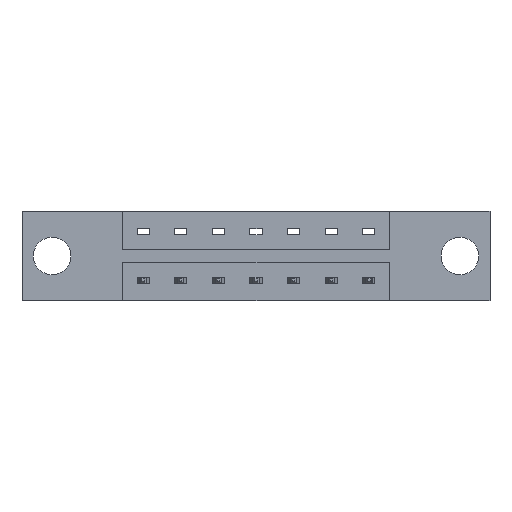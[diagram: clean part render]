
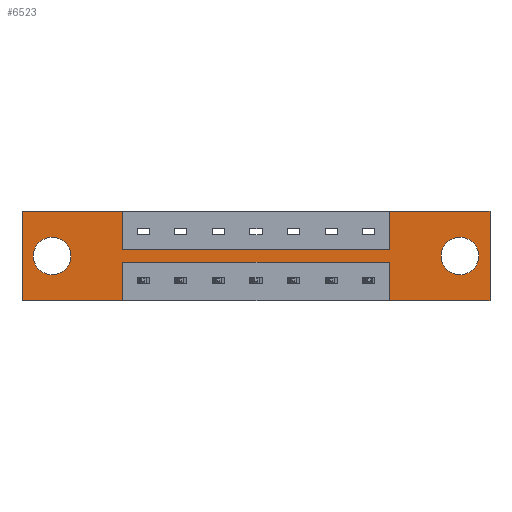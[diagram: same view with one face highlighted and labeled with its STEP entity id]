
A CAD part, front view. The second image highlights one B-rep face of the part: STEP entity #6523.
In plain terms, the highlighted planar face has unit normal (0, -1, 0).
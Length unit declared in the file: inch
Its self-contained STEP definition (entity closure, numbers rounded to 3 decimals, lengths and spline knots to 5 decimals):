
#17 = VECTOR ( 'NONE', #7473, 39.37008 ) ;
#23 = ORIENTED_EDGE ( 'NONE', *, *, #1032, .F. ) ;
#30 = ORIENTED_EDGE ( 'NONE', *, *, #563, .F. ) ;
#57 = ORIENTED_EDGE ( 'NONE', *, *, #378, .F. ) ;
#73 = ORIENTED_EDGE ( 'NONE', *, *, #656, .F. ) ;
#110 = ORIENTED_EDGE ( 'NONE', *, *, #6834, .T. ) ;
#120 = ORIENTED_EDGE ( 'NONE', *, *, #4638, .T. ) ;
#165 = ORIENTED_EDGE ( 'NONE', *, *, #4374, .T. ) ;
#191 = VECTOR ( 'NONE', #8565, 39.37008 ) ;
#202 = ORIENTED_EDGE ( 'NONE', *, *, #7367, .T. ) ;
#263 = LINE ( 'NONE', #601, #5720 ) ;
#378 = EDGE_CURVE ( 'NONE', #4003, #1568, #4932, .T. ) ;
#405 = DIRECTION ( 'NONE',  ( -1., 0., 0. ) ) ;
#531 = VERTEX_POINT ( 'NONE', #6383 ) ;
#543 = ORIENTED_EDGE ( 'NONE', *, *, #3752, .F. ) ;
#558 = CARTESIAN_POINT ( 'NONE',  ( 0., 0., -0.37 ) ) ;
#563 = EDGE_CURVE ( 'NONE', #1877, #4003, #7671, .T. ) ;
#576 = CARTESIAN_POINT ( 'NONE',  ( 0., 0., -0.37 ) ) ;
#601 = CARTESIAN_POINT ( 'NONE',  ( 0.4175, 0., -0.1585 ) ) ;
#637 = DIRECTION ( 'NONE',  ( 0., 0., -1. ) ) ;
#656 = EDGE_CURVE ( 'NONE', #1568, #5507, #3404, .T. ) ;
#722 = EDGE_CURVE ( 'NONE', #6039, #4532, #4184, .T. ) ;
#800 = CIRCLE ( 'NONE', #4775, 0.078 ) ;
#1019 = EDGE_CURVE ( 'NONE', #4742, #1957, #5601, .T. ) ;
#1032 = EDGE_CURVE ( 'NONE', #7844, #1877, #7390, .T. ) ;
#1098 = DIRECTION ( 'NONE',  ( 0., 1., 0. ) ) ;
#1151 = CARTESIAN_POINT ( 'NONE',  ( 0., 0., -0.37 ) ) ;
#1164 = VERTEX_POINT ( 'NONE', #2312 ) ;
#1307 = CARTESIAN_POINT ( 'NONE',  ( 0., 0., 0. ) ) ;
#1497 = LINE ( 'NONE', #8006, #8509 ) ;
#1498 = EDGE_LOOP ( 'NONE', ( #120, #110 ) ) ;
#1534 = CARTESIAN_POINT ( 'NONE',  ( 0., 0., 0. ) ) ;
#1568 = VERTEX_POINT ( 'NONE', #5871 ) ;
#1825 = VECTOR ( 'NONE', #7813, 39.37008 ) ;
#1860 = ORIENTED_EDGE ( 'NONE', *, *, #6313, .F. ) ;
#1877 = VERTEX_POINT ( 'NONE', #8606 ) ;
#1878 = ORIENTED_EDGE ( 'NONE', *, *, #1019, .F. ) ;
#1957 = VERTEX_POINT ( 'NONE', #7515 ) ;
#2075 = CARTESIAN_POINT ( 'NONE',  ( 0., 0., -0.37 ) ) ;
#2192 = VECTOR ( 'NONE', #3159, 39.37008 ) ;
#2207 = DIRECTION ( 'NONE',  ( -1., 0., 0. ) ) ;
#2263 = VECTOR ( 'NONE', #4279, 39.37008 ) ;
#2283 = ORIENTED_EDGE ( 'NONE', *, *, #7035, .F. ) ;
#2312 = CARTESIAN_POINT ( 'NONE',  ( 1.815, 0., -0.263 ) ) ;
#2666 = VECTOR ( 'NONE', #4414, 39.37008 ) ;
#2792 = DIRECTION ( 'NONE',  ( 1., 0., 0. ) ) ;
#2845 = VECTOR ( 'NONE', #3826, 39.37008 ) ;
#2872 = CARTESIAN_POINT ( 'NONE',  ( 0.125, 0., -0.185 ) ) ;
#3081 = VECTOR ( 'NONE', #2207, 39.37008 ) ;
#3150 = VERTEX_POINT ( 'NONE', #6538 ) ;
#3158 = EDGE_CURVE ( 'NONE', #1957, #5408, #7629, .T. ) ;
#3159 = DIRECTION ( 'NONE',  ( 0., 0., -1. ) ) ;
#3190 = DIRECTION ( 'NONE',  ( 0., 1., 0. ) ) ;
#3228 = CARTESIAN_POINT ( 'NONE',  ( 1.5225, 0., -0.1585 ) ) ;
#3303 = FACE_OUTER_BOUND ( 'NONE', #4611, .T. ) ;
#3325 = CARTESIAN_POINT ( 'NONE',  ( 0.4175, 0., -0.2115 ) ) ;
#3389 = DIRECTION ( 'NONE',  ( 1., 0., 0. ) ) ;
#3404 = LINE ( 'NONE', #8135, #8120 ) ;
#3505 = CARTESIAN_POINT ( 'NONE',  ( 1.94, 0., -0.37 ) ) ;
#3581 = DIRECTION ( 'NONE',  ( 0., 0., 1. ) ) ;
#3752 = EDGE_CURVE ( 'NONE', #7114, #7844, #6810, .T. ) ;
#3754 = CARTESIAN_POINT ( 'NONE',  ( 0.125, 0., -0.107 ) ) ;
#3820 = EDGE_CURVE ( 'NONE', #3150, #6039, #7707, .T. ) ;
#3826 = DIRECTION ( 'NONE',  ( 0., 0., 1. ) ) ;
#3873 = CARTESIAN_POINT ( 'NONE',  ( 1.5225, 0., -0.2115 ) ) ;
#3943 = ORIENTED_EDGE ( 'NONE', *, *, #5784, .F. ) ;
#3980 = AXIS2_PLACEMENT_3D ( 'NONE', #8790, #4918, #637 ) ;
#4003 = VERTEX_POINT ( 'NONE', #3505 ) ;
#4110 = AXIS2_PLACEMENT_3D ( 'NONE', #2872, #7662, #3581 ) ;
#4184 = LINE ( 'NONE', #1151, #2263 ) ;
#4257 = PLANE ( 'NONE',  #5407 ) ;
#4279 = DIRECTION ( 'NONE',  ( -1., 0., 0. ) ) ;
#4374 = EDGE_CURVE ( 'NONE', #1164, #531, #6489, .T. ) ;
#4414 = DIRECTION ( 'NONE',  ( 0., 0., 1. ) ) ;
#4532 = VERTEX_POINT ( 'NONE', #558 ) ;
#4581 = CARTESIAN_POINT ( 'NONE',  ( 1.94, 0., 0. ) ) ;
#4611 = EDGE_LOOP ( 'NONE', ( #73, #57, #30, #23, #543, #3943, #6096, #1878, #2283, #7335, #6773, #1860 ) ) ;
#4630 = AXIS2_PLACEMENT_3D ( 'NONE', #5359, #1098, #6067 ) ;
#4638 = EDGE_CURVE ( 'NONE', #6944, #6542, #5943, .T. ) ;
#4742 = VERTEX_POINT ( 'NONE', #1534 ) ;
#4775 = AXIS2_PLACEMENT_3D ( 'NONE', #7309, #3190, #7923 ) ;
#4849 = CARTESIAN_POINT ( 'NONE',  ( 1.5225, 0., -0.1585 ) ) ;
#4918 = DIRECTION ( 'NONE',  ( 0., 1., 0. ) ) ;
#4925 = DIRECTION ( 'NONE',  ( 0., 0., -1. ) ) ;
#4932 = LINE ( 'NONE', #576, #3081 ) ;
#5122 = CARTESIAN_POINT ( 'NONE',  ( 0.4175, 0., -0.37 ) ) ;
#5142 = CIRCLE ( 'NONE', #3980, 0.078 ) ;
#5160 = FACE_BOUND ( 'NONE', #1498, .T. ) ;
#5359 = CARTESIAN_POINT ( 'NONE',  ( 1.815, 0., -0.185 ) ) ;
#5407 = AXIS2_PLACEMENT_3D ( 'NONE', #2075, #8797, #4925 ) ;
#5408 = VERTEX_POINT ( 'NONE', #7195 ) ;
#5507 = VERTEX_POINT ( 'NONE', #3873 ) ;
#5601 = LINE ( 'NONE', #6052, #8779 ) ;
#5720 = VECTOR ( 'NONE', #2792, 39.37008 ) ;
#5784 = EDGE_CURVE ( 'NONE', #5408, #7114, #263, .T. ) ;
#5871 = CARTESIAN_POINT ( 'NONE',  ( 1.5225, 0., -0.37 ) ) ;
#5943 = CIRCLE ( 'NONE', #4110, 0.078 ) ;
#6039 = VERTEX_POINT ( 'NONE', #5122 ) ;
#6050 = CARTESIAN_POINT ( 'NONE',  ( 1.5225, 0., 0. ) ) ;
#6052 = CARTESIAN_POINT ( 'NONE',  ( 0., 0., 0. ) ) ;
#6067 = DIRECTION ( 'NONE',  ( 0., 0., -1. ) ) ;
#6096 = ORIENTED_EDGE ( 'NONE', *, *, #3158, .F. ) ;
#6119 = EDGE_LOOP ( 'NONE', ( #202, #165 ) ) ;
#6313 = EDGE_CURVE ( 'NONE', #5507, #3150, #1497, .T. ) ;
#6383 = CARTESIAN_POINT ( 'NONE',  ( 1.815, 0., -0.107 ) ) ;
#6489 = CIRCLE ( 'NONE', #4630, 0.078 ) ;
#6523 = ADVANCED_FACE ( 'NONE', ( #6771, #5160, #3303 ), #4257, .T. ) ;
#6538 = CARTESIAN_POINT ( 'NONE',  ( 0.4175, 0., -0.2115 ) ) ;
#6542 = VERTEX_POINT ( 'NONE', #8826 ) ;
#6554 = LINE ( 'NONE', #6592, #2845 ) ;
#6592 = CARTESIAN_POINT ( 'NONE',  ( 0., 0., 0. ) ) ;
#6771 = FACE_BOUND ( 'NONE', #6119, .T. ) ;
#6773 = ORIENTED_EDGE ( 'NONE', *, *, #3820, .F. ) ;
#6810 = LINE ( 'NONE', #4849, #2666 ) ;
#6834 = EDGE_CURVE ( 'NONE', #6542, #6944, #800, .T. ) ;
#6941 = CARTESIAN_POINT ( 'NONE',  ( 0.4175, 0., -0.1585 ) ) ;
#6944 = VERTEX_POINT ( 'NONE', #3754 ) ;
#7035 = EDGE_CURVE ( 'NONE', #4532, #4742, #6554, .T. ) ;
#7114 = VERTEX_POINT ( 'NONE', #3228 ) ;
#7195 = CARTESIAN_POINT ( 'NONE',  ( 0.4175, 0., -0.1585 ) ) ;
#7309 = CARTESIAN_POINT ( 'NONE',  ( 0.125, 0., -0.185 ) ) ;
#7335 = ORIENTED_EDGE ( 'NONE', *, *, #722, .F. ) ;
#7367 = EDGE_CURVE ( 'NONE', #531, #1164, #5142, .T. ) ;
#7390 = LINE ( 'NONE', #1307, #1825 ) ;
#7473 = DIRECTION ( 'NONE',  ( 0., 0., -1. ) ) ;
#7515 = CARTESIAN_POINT ( 'NONE',  ( 0.4175, 0., 0. ) ) ;
#7629 = LINE ( 'NONE', #6941, #191 ) ;
#7662 = DIRECTION ( 'NONE',  ( 0., 1., 0. ) ) ;
#7671 = LINE ( 'NONE', #4581, #17 ) ;
#7707 = LINE ( 'NONE', #3325, #2192 ) ;
#7813 = DIRECTION ( 'NONE',  ( 1., 0., 0. ) ) ;
#7844 = VERTEX_POINT ( 'NONE', #6050 ) ;
#7923 = DIRECTION ( 'NONE',  ( 0., 0., 1. ) ) ;
#8006 = CARTESIAN_POINT ( 'NONE',  ( 0.4175, 0., -0.2115 ) ) ;
#8120 = VECTOR ( 'NONE', #8160, 39.37008 ) ;
#8135 = CARTESIAN_POINT ( 'NONE',  ( 1.5225, 0., -0.2115 ) ) ;
#8160 = DIRECTION ( 'NONE',  ( 0., 0., 1. ) ) ;
#8509 = VECTOR ( 'NONE', #405, 39.37008 ) ;
#8565 = DIRECTION ( 'NONE',  ( 0., 0., -1. ) ) ;
#8606 = CARTESIAN_POINT ( 'NONE',  ( 1.94, 0., 0. ) ) ;
#8779 = VECTOR ( 'NONE', #3389, 39.37008 ) ;
#8790 = CARTESIAN_POINT ( 'NONE',  ( 1.815, 0., -0.185 ) ) ;
#8797 = DIRECTION ( 'NONE',  ( 0., -1., 0. ) ) ;
#8826 = CARTESIAN_POINT ( 'NONE',  ( 0.125, 0., -0.263 ) ) ;
